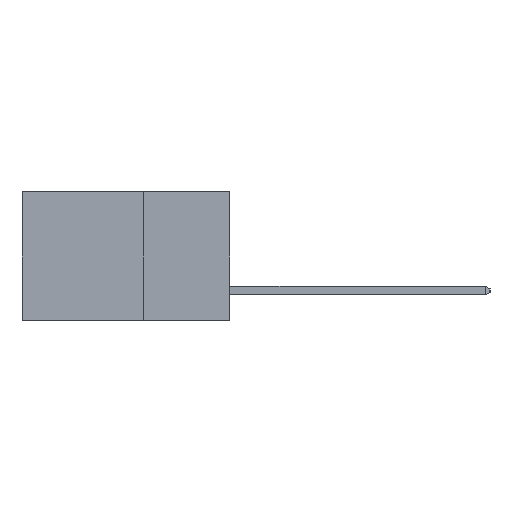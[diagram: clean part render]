
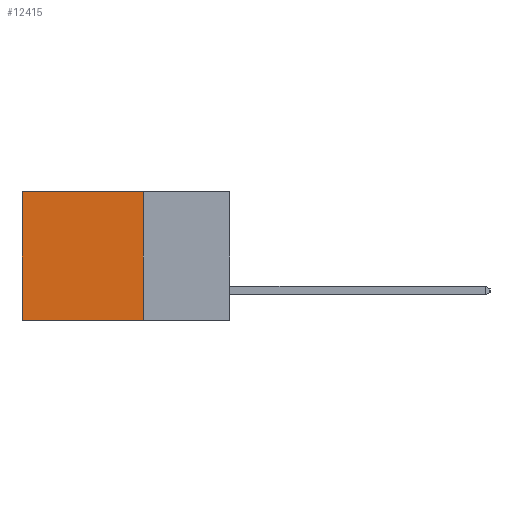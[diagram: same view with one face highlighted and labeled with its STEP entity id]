
A CAD part, left-side view. The second image highlights one B-rep face of the part: STEP entity #12415.
In plain terms, the highlighted planar face has unit normal (-1, 0, 0).
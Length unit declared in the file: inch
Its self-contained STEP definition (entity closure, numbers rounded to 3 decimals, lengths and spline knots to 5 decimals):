
#16 = PLANE ( 'NONE',  #3048 ) ;
#57 = ORIENTED_EDGE ( 'NONE', *, *, #283, .T. ) ;
#283 = EDGE_CURVE ( 'NONE', #6290, #8836, #1586, .T. ) ;
#784 = ORIENTED_EDGE ( 'NONE', *, *, #6087, .T. ) ;
#1035 = EDGE_LOOP ( 'NONE', ( #784, #9556, #11201, #57 ) ) ;
#1073 = VECTOR ( 'NONE', #1970, 39.37008 ) ;
#1586 = LINE ( 'NONE', #8631, #4074 ) ;
#1823 = CARTESIAN_POINT ( 'NONE',  ( 0.2615, 0.6, -0.37 ) ) ;
#1970 = DIRECTION ( 'NONE',  ( 0., 0., -1. ) ) ;
#1975 = CARTESIAN_POINT ( 'NONE',  ( 0.2615, 0.25, 0. ) ) ;
#2016 = CARTESIAN_POINT ( 'NONE',  ( 0.2615, 0.6, -0.37 ) ) ;
#2822 = VECTOR ( 'NONE', #3377, 39.37008 ) ;
#3048 = AXIS2_PLACEMENT_3D ( 'NONE', #3323, #10023, #4356 ) ;
#3323 = CARTESIAN_POINT ( 'NONE',  ( 0.2615, 0.25, -0.37 ) ) ;
#3377 = DIRECTION ( 'NONE',  ( 0., 1., 0. ) ) ;
#3529 = CARTESIAN_POINT ( 'NONE',  ( 0.2615, 0.25, -0.37 ) ) ;
#3826 = CARTESIAN_POINT ( 'NONE',  ( 0.2615, 0.25, -0.37 ) ) ;
#4074 = VECTOR ( 'NONE', #7270, 39.37008 ) ;
#4356 = DIRECTION ( 'NONE',  ( 0., 0., -1. ) ) ;
#5472 = LINE ( 'NONE', #3529, #2822 ) ;
#5944 = EDGE_CURVE ( 'NONE', #8714, #9341, #5472, .T. ) ;
#6087 = EDGE_CURVE ( 'NONE', #8836, #9341, #11780, .T. ) ;
#6290 = VERTEX_POINT ( 'NONE', #1975 ) ;
#6738 = EDGE_CURVE ( 'NONE', #6290, #8714, #7345, .T. ) ;
#7270 = DIRECTION ( 'NONE',  ( 0., 1., 0. ) ) ;
#7345 = LINE ( 'NONE', #3826, #7660 ) ;
#7660 = VECTOR ( 'NONE', #10462, 39.37008 ) ;
#8074 = CARTESIAN_POINT ( 'NONE',  ( 0.2615, 0.6, 0. ) ) ;
#8631 = CARTESIAN_POINT ( 'NONE',  ( 0.2615, 0.25, 0. ) ) ;
#8714 = VERTEX_POINT ( 'NONE', #11672 ) ;
#8836 = VERTEX_POINT ( 'NONE', #8074 ) ;
#9341 = VERTEX_POINT ( 'NONE', #1823 ) ;
#9556 = ORIENTED_EDGE ( 'NONE', *, *, #5944, .F. ) ;
#9745 = FACE_OUTER_BOUND ( 'NONE', #1035, .T. ) ;
#10023 = DIRECTION ( 'NONE',  ( 1., 0., 0. ) ) ;
#10462 = DIRECTION ( 'NONE',  ( 0., 0., -1. ) ) ;
#11201 = ORIENTED_EDGE ( 'NONE', *, *, #6738, .F. ) ;
#11672 = CARTESIAN_POINT ( 'NONE',  ( 0.2615, 0.25, -0.37 ) ) ;
#11780 = LINE ( 'NONE', #2016, #1073 ) ;
#12415 = ADVANCED_FACE ( 'NONE', ( #9745 ), #16, .F. ) ;
